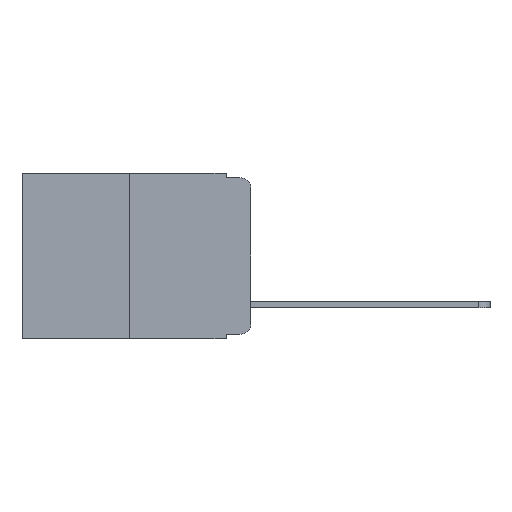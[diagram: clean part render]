
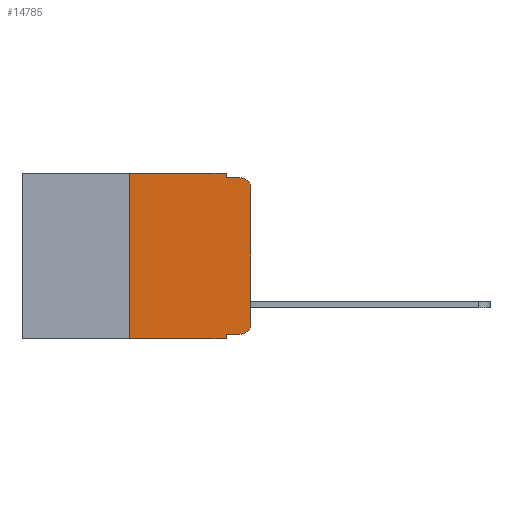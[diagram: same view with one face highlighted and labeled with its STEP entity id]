
A CAD part, left-side view. The second image highlights one B-rep face of the part: STEP entity #14785.
In plain terms, the highlighted planar face has unit normal (-1, 0, 0).
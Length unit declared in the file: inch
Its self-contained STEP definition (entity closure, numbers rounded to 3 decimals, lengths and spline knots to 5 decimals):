
#43 = VECTOR ( 'NONE', #18743, 39.37008 ) ;
#596 = LINE ( 'NONE', #18330, #19328 ) ;
#678 = CARTESIAN_POINT ( 'NONE',  ( 0., 0.051, -0.01 ) ) ;
#912 = VECTOR ( 'NONE', #12113, 39.37008 ) ;
#1973 = EDGE_CURVE ( 'NONE', #17412, #21032, #3867, .T. ) ;
#2103 = CARTESIAN_POINT ( 'NONE',  ( 0., 0.051, 0. ) ) ;
#2242 = VERTEX_POINT ( 'NONE', #2393 ) ;
#2393 = CARTESIAN_POINT ( 'NONE',  ( 0., 0.25, -0.343 ) ) ;
#2543 = EDGE_CURVE ( 'NONE', #2242, #13144, #11206, .T. ) ;
#2648 = LINE ( 'NONE', #5167, #7868 ) ;
#3522 = EDGE_LOOP ( 'NONE', ( #18932, #7304, #9965, #11238, #12101, #3725, #17326, #12631, #10142, #22171 ) ) ;
#3725 = ORIENTED_EDGE ( 'NONE', *, *, #2543, .F. ) ;
#3867 = CIRCLE ( 'NONE', #11710, 0.02 ) ;
#4181 = DIRECTION ( 'NONE',  ( 0., -1., 0. ) ) ;
#4634 = CARTESIAN_POINT ( 'NONE',  ( 0., 0.051, -0.343 ) ) ;
#5140 = LINE ( 'NONE', #16094, #10309 ) ;
#5167 = CARTESIAN_POINT ( 'NONE',  ( 0., 0.473, 0. ) ) ;
#5196 = CARTESIAN_POINT ( 'NONE',  ( 0., 0.02, -0.333 ) ) ;
#5552 = DIRECTION ( 'NONE',  ( 0., -1., 0. ) ) ;
#5931 = DIRECTION ( 'NONE',  ( 0., 0., -1. ) ) ;
#6086 = CARTESIAN_POINT ( 'NONE',  ( 0., 0.051, 0. ) ) ;
#6288 = EDGE_CURVE ( 'NONE', #16940, #18679, #15512, .T. ) ;
#6291 = VECTOR ( 'NONE', #5931, 39.37008 ) ;
#6581 = VECTOR ( 'NONE', #22458, 39.37008 ) ;
#6597 = CARTESIAN_POINT ( 'NONE',  ( 0., 0.473, 0. ) ) ;
#7304 = ORIENTED_EDGE ( 'NONE', *, *, #1973, .T. ) ;
#7353 = EDGE_CURVE ( 'NONE', #2242, #8476, #596, .T. ) ;
#7868 = VECTOR ( 'NONE', #20901, 39.37008 ) ;
#7895 = EDGE_CURVE ( 'NONE', #21738, #16940, #17101, .T. ) ;
#8167 = DIRECTION ( 'NONE',  ( 0., 0., -1. ) ) ;
#8338 = LINE ( 'NONE', #15778, #912 ) ;
#8476 = VERTEX_POINT ( 'NONE', #4634 ) ;
#8686 = VERTEX_POINT ( 'NONE', #678 ) ;
#8847 = FACE_OUTER_BOUND ( 'NONE', #3522, .T. ) ;
#9229 = DIRECTION ( 'NONE',  ( 0., 0., -1. ) ) ;
#9965 = ORIENTED_EDGE ( 'NONE', *, *, #11636, .F. ) ;
#10142 = ORIENTED_EDGE ( 'NONE', *, *, #7895, .T. ) ;
#10309 = VECTOR ( 'NONE', #5552, 39.37008 ) ;
#10927 = LINE ( 'NONE', #6086, #6291 ) ;
#11206 = LINE ( 'NONE', #18770, #6581 ) ;
#11238 = ORIENTED_EDGE ( 'NONE', *, *, #15307, .F. ) ;
#11636 = EDGE_CURVE ( 'NONE', #8686, #21032, #5140, .T. ) ;
#11710 = AXIS2_PLACEMENT_3D ( 'NONE', #15215, #16973, #8167 ) ;
#11718 = CARTESIAN_POINT ( 'NONE',  ( 0., 0.02, -0.313 ) ) ;
#12101 = ORIENTED_EDGE ( 'NONE', *, *, #21955, .F. ) ;
#12113 = DIRECTION ( 'NONE',  ( 0., 0., 1. ) ) ;
#12116 = VECTOR ( 'NONE', #9229, 39.37008 ) ;
#12473 = EDGE_CURVE ( 'NONE', #18679, #17412, #8338, .T. ) ;
#12631 = ORIENTED_EDGE ( 'NONE', *, *, #21079, .F. ) ;
#13144 = VERTEX_POINT ( 'NONE', #13971 ) ;
#13336 = VERTEX_POINT ( 'NONE', #2103 ) ;
#13971 = CARTESIAN_POINT ( 'NONE',  ( 0., 0.25, 0. ) ) ;
#14542 = AXIS2_PLACEMENT_3D ( 'NONE', #6597, #20577, #18653 ) ;
#14769 = CARTESIAN_POINT ( 'NONE',  ( 0., 0.051, -0.333 ) ) ;
#14785 = ADVANCED_FACE ( 'NONE', ( #8847 ), #17146, .F. ) ;
#15215 = CARTESIAN_POINT ( 'NONE',  ( 0., 0.02, -0.03 ) ) ;
#15307 = EDGE_CURVE ( 'NONE', #13336, #8686, #19823, .T. ) ;
#15512 = CIRCLE ( 'NONE', #18377, 0.02 ) ;
#15778 = CARTESIAN_POINT ( 'NONE',  ( 0., 0., 0. ) ) ;
#16094 = CARTESIAN_POINT ( 'NONE',  ( 0., 0.051, -0.01 ) ) ;
#16264 = CARTESIAN_POINT ( 'NONE',  ( 0., 0.051, 0. ) ) ;
#16766 = CARTESIAN_POINT ( 'NONE',  ( 0., 0.051, -0.333 ) ) ;
#16852 = DIRECTION ( 'NONE',  ( 0., 0., -1. ) ) ;
#16940 = VERTEX_POINT ( 'NONE', #5196 ) ;
#16973 = DIRECTION ( 'NONE',  ( -1., 0., 0. ) ) ;
#17101 = LINE ( 'NONE', #14769, #43 ) ;
#17146 = PLANE ( 'NONE',  #14542 ) ;
#17326 = ORIENTED_EDGE ( 'NONE', *, *, #7353, .T. ) ;
#17412 = VERTEX_POINT ( 'NONE', #20145 ) ;
#18330 = CARTESIAN_POINT ( 'NONE',  ( 0., 0.473, -0.343 ) ) ;
#18377 = AXIS2_PLACEMENT_3D ( 'NONE', #11718, #20517, #16852 ) ;
#18653 = DIRECTION ( 'NONE',  ( 0., 0., -1. ) ) ;
#18679 = VERTEX_POINT ( 'NONE', #20859 ) ;
#18743 = DIRECTION ( 'NONE',  ( 0., -1., 0. ) ) ;
#18770 = CARTESIAN_POINT ( 'NONE',  ( 0., 0.25, 0. ) ) ;
#18932 = ORIENTED_EDGE ( 'NONE', *, *, #12473, .T. ) ;
#19328 = VECTOR ( 'NONE', #4181, 39.37008 ) ;
#19823 = LINE ( 'NONE', #16264, #12116 ) ;
#20145 = CARTESIAN_POINT ( 'NONE',  ( 0., 0., -0.03 ) ) ;
#20517 = DIRECTION ( 'NONE',  ( -1., 0., 0. ) ) ;
#20577 = DIRECTION ( 'NONE',  ( 1., 0., 0. ) ) ;
#20859 = CARTESIAN_POINT ( 'NONE',  ( 0., 0., -0.313 ) ) ;
#20901 = DIRECTION ( 'NONE',  ( 0., -1., 0. ) ) ;
#21032 = VERTEX_POINT ( 'NONE', #21746 ) ;
#21079 = EDGE_CURVE ( 'NONE', #21738, #8476, #10927, .T. ) ;
#21738 = VERTEX_POINT ( 'NONE', #16766 ) ;
#21746 = CARTESIAN_POINT ( 'NONE',  ( 0., 0.02, -0.01 ) ) ;
#21955 = EDGE_CURVE ( 'NONE', #13144, #13336, #2648, .T. ) ;
#22171 = ORIENTED_EDGE ( 'NONE', *, *, #6288, .T. ) ;
#22458 = DIRECTION ( 'NONE',  ( 0., 0., 1. ) ) ;
